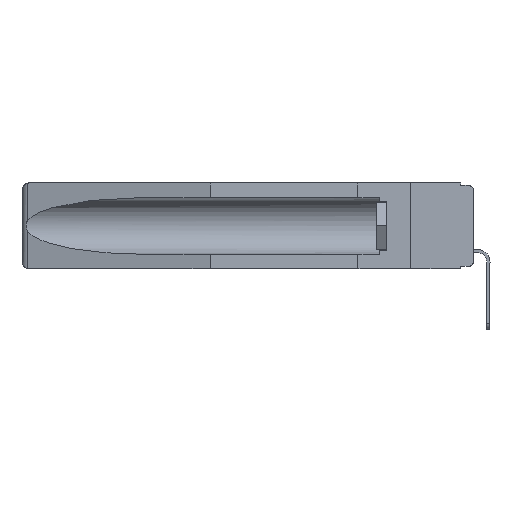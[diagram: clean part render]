
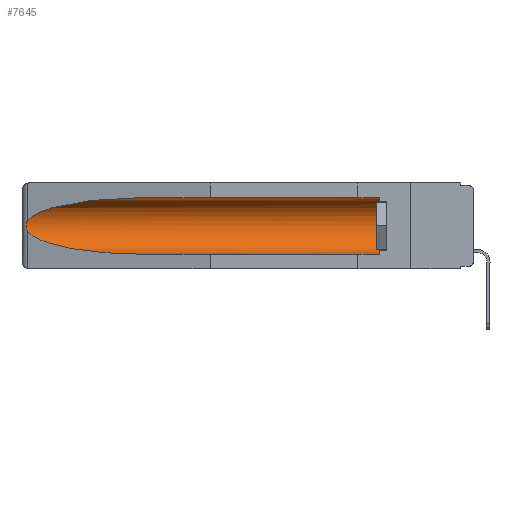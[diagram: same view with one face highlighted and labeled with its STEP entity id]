
A CAD part, left-side view. The second image highlights one B-rep face of the part: STEP entity #7645.
In plain terms, the highlighted cylindrical face has radius 2.857 mm (diameter 5.715 mm), a partial arc.
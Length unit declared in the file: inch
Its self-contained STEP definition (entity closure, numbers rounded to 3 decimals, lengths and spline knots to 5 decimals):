
#110 = EDGE_CURVE ( 'NONE', #4925, #1290, #10151, .T. ) ;
#342 = CARTESIAN_POINT ( 'NONE',  ( 0.155, -0.30754, -0.1715 ) ) ;
#420 = CARTESIAN_POINT ( 'NONE',  ( 0.21114, 1.30732, -0.284 ) ) ;
#627 = VECTOR ( 'NONE', #14841, 39.37008 ) ;
#1290 = VERTEX_POINT ( 'NONE', #13409 ) ;
#1494 = CARTESIAN_POINT ( 'NONE',  ( 0.155, 0.126, -0.1715 ) ) ;
#1910 = CARTESIAN_POINT ( 'NONE',  ( 0.26537, 1.52718, -0.19328 ) ) ;
#2141 = VECTOR ( 'NONE', #4760, 39.37008 ) ;
#3030 = LINE ( 'NONE', #5829, #2141 ) ;
#3123 = CARTESIAN_POINT ( 'NONE',  ( 0.2675, 1.53308, -0.16763 ) ) ;
#3441 = DIRECTION ( 'NONE',  ( 0., 1., 0. ) ) ;
#3625 = EDGE_CURVE ( 'NONE', #6748, #17307, #17133, .T. ) ;
#4480 = CARTESIAN_POINT ( 'NONE',  ( 0.26537, 1.52718, -0.19328 ) ) ;
#4760 = DIRECTION ( 'NONE',  ( 0., 1., 0. ) ) ;
#4925 = VERTEX_POINT ( 'NONE', #12611 ) ;
#5158 = ORIENTED_EDGE ( 'NONE', *, *, #110, .T. ) ;
#5269 = CARTESIAN_POINT ( 'NONE',  ( 0.155, 1.07973, -0.059 ) ) ;
#5829 = CARTESIAN_POINT ( 'NONE',  ( 0.155, -0.30754, -0.284 ) ) ;
#5894 = CARTESIAN_POINT ( 'NONE',  ( 0.155, 1.07973, -0.284 ) ) ;
#5922 = EDGE_CURVE ( 'NONE', #17307, #4925, #10629, .T. ) ;
#5925 = CARTESIAN_POINT ( 'NONE',  ( 0.26537, 1.52718, -0.14972 ) ) ;
#6011 = CARTESIAN_POINT ( 'NONE',  ( 0.26654, 1.53092, -0.15636 ) ) ;
#6127 = CARTESIAN_POINT ( 'NONE',  ( 0.155, 1.07973, -0.284 ) ) ;
#6748 = VERTEX_POINT ( 'NONE', #17541 ) ;
#7066 = CARTESIAN_POINT ( 'NONE',  ( 0.155, 0.126, -0.059 ) ) ;
#7109 = CARTESIAN_POINT ( 'NONE',  ( 0.26597, 1.5296, -0.19026 ) ) ;
#7645 = ADVANCED_FACE ( 'NONE', ( #14475 ), #13177, .F. ) ;
#8073 = CARTESIAN_POINT ( 'NONE',  ( 0.26537, 1.52718, -0.14972 ) ) ;
#8161 = CARTESIAN_POINT ( 'NONE',  ( 0.21114, 1.30732, -0.059 ) ) ;
#8666 = CARTESIAN_POINT ( 'NONE',  ( 0.2673, 1.53269, -0.17917 ) ) ;
#8707 = DIRECTION ( 'NONE',  ( 0., 0., 1. ) ) ;
#9187 = CARTESIAN_POINT ( 'NONE',  ( 0.25451, 1.48313, -0.09465 ) ) ;
#9189 = ORIENTED_EDGE ( 'NONE', *, *, #5922, .T. ) ;
#9251 = AXIS2_PLACEMENT_3D ( 'NONE', #1494, #15282, #11142 ) ;
#9301 = EDGE_LOOP ( 'NONE', ( #5158, #11795, #16780, #15480, #13245, #9189 ) ) ;
#9476 =( BOUNDED_CURVE ( )  B_SPLINE_CURVE ( 3, ( #10153, #12977, #420, #6127 ),
 .UNSPECIFIED., .F., .T. ) 
 B_SPLINE_CURVE_WITH_KNOTS ( ( 4, 4 ),
 ( 0.1948, 1.5708 ),
 .UNSPECIFIED. ) 
 CURVE ( )  GEOMETRIC_REPRESENTATION_ITEM ( )  RATIONAL_B_SPLINE_CURVE ( ( 1., 0.848, 0.848, 1. ) ) 
 REPRESENTATION_ITEM ( '' )  );
#10151 =( BOUNDED_CURVE ( )  B_SPLINE_CURVE ( 3, ( #5269, #8161, #9187, #8073 ),
 .UNSPECIFIED., .F., .T. ) 
 B_SPLINE_CURVE_WITH_KNOTS ( ( 4, 4 ),
 ( 4.71239, 6.08839 ),
 .UNSPECIFIED. ) 
 CURVE ( )  GEOMETRIC_REPRESENTATION_ITEM ( )  RATIONAL_B_SPLINE_CURVE ( ( 1., 0.848, 0.848, 1. ) ) 
 REPRESENTATION_ITEM ( '' )  );
#10153 = CARTESIAN_POINT ( 'NONE',  ( 0.26537, 1.52718, -0.19328 ) ) ;
#10285 = AXIS2_PLACEMENT_3D ( 'NONE', #342, #3441, #8707 ) ;
#10442 = CARTESIAN_POINT ( 'NONE',  ( 0.155, -0.30754, -0.059 ) ) ;
#10629 = LINE ( 'NONE', #10442, #627 ) ;
#11142 = DIRECTION ( 'NONE',  ( 0., 0., 1. ) ) ;
#11398 = CARTESIAN_POINT ( 'NONE',  ( 0.26597, 1.52961, -0.15275 ) ) ;
#11402 = B_SPLINE_CURVE_WITH_KNOTS ( 'NONE', 3,
 ( #5925, #11398, #6011, #11591, #3123, #15724, #8666, #12954, #7109, #4480 ),
 .UNSPECIFIED., .F., .F.,
 ( 4, 2, 2, 2, 4 ),
 ( 0., 0.00029, 0.00058, 0.00087, 0.00117 ),
 .UNSPECIFIED. ) ;
#11558 = VERTEX_POINT ( 'NONE', #5894 ) ;
#11591 = CARTESIAN_POINT ( 'NONE',  ( 0.2673, 1.5327, -0.16383 ) ) ;
#11795 = ORIENTED_EDGE ( 'NONE', *, *, #13207, .T. ) ;
#12611 = CARTESIAN_POINT ( 'NONE',  ( 0.155, 1.07973, -0.059 ) ) ;
#12954 = CARTESIAN_POINT ( 'NONE',  ( 0.26655, 1.53094, -0.18657 ) ) ;
#12977 = CARTESIAN_POINT ( 'NONE',  ( 0.25451, 1.48313, -0.24835 ) ) ;
#13177 = CYLINDRICAL_SURFACE ( 'NONE', #10285, 0.1125 ) ;
#13207 = EDGE_CURVE ( 'NONE', #1290, #14857, #11402, .T. ) ;
#13245 = ORIENTED_EDGE ( 'NONE', *, *, #3625, .T. ) ;
#13409 = CARTESIAN_POINT ( 'NONE',  ( 0.26537, 1.52718, -0.14972 ) ) ;
#14036 = EDGE_CURVE ( 'NONE', #14857, #11558, #9476, .T. ) ;
#14475 = FACE_OUTER_BOUND ( 'NONE', #9301, .T. ) ;
#14552 = EDGE_CURVE ( 'NONE', #6748, #11558, #3030, .T. ) ;
#14841 = DIRECTION ( 'NONE',  ( 0., 1., 0. ) ) ;
#14857 = VERTEX_POINT ( 'NONE', #1910 ) ;
#15282 = DIRECTION ( 'NONE',  ( 0., -1., 0. ) ) ;
#15480 = ORIENTED_EDGE ( 'NONE', *, *, #14552, .F. ) ;
#15724 = CARTESIAN_POINT ( 'NONE',  ( 0.2675, 1.53308, -0.17534 ) ) ;
#16780 = ORIENTED_EDGE ( 'NONE', *, *, #14036, .T. ) ;
#17133 = CIRCLE ( 'NONE', #9251, 0.1125 ) ;
#17307 = VERTEX_POINT ( 'NONE', #7066 ) ;
#17541 = CARTESIAN_POINT ( 'NONE',  ( 0.155, 0.126, -0.284 ) ) ;
